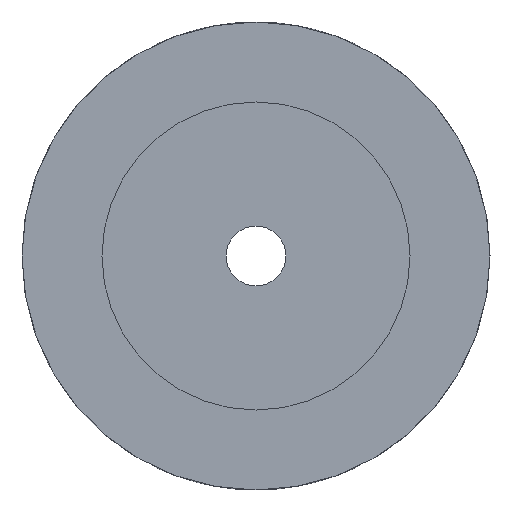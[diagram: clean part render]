
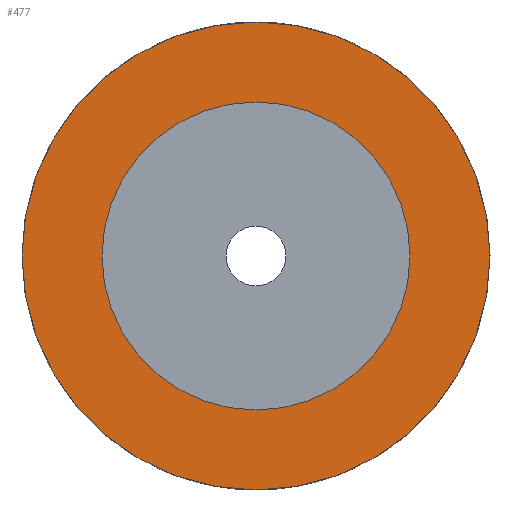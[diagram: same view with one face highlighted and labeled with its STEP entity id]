
A CAD part, front view. The second image highlights one B-rep face of the part: STEP entity #477.
In plain terms, the highlighted planar face has unit normal (0, -1, 0).
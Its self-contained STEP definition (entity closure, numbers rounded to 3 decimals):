
#27 = CARTESIAN_POINT ( 'NONE',  ( -2.625, 5.715, 0. ) ) ;
#30 = DIRECTION ( 'NONE',  ( -1., 0., 0. ) ) ;
#31 = DIRECTION ( 'NONE',  ( 0., 1., 0. ) ) ;
#33 = CARTESIAN_POINT ( 'NONE',  ( 0., 5.715, 0. ) ) ;
#34 = PLANE ( 'NONE',  #389 ) ;
#35 = CARTESIAN_POINT ( 'NONE',  ( 2.625, 5.715, 0. ) ) ;
#53 = CARTESIAN_POINT ( 'NONE',  ( -3.988, 5.715, 0. ) ) ;
#84 = DIRECTION ( 'NONE',  ( -1., 0., 0. ) ) ;
#85 = DIRECTION ( 'NONE',  ( 0., 1., 0. ) ) ;
#86 = CARTESIAN_POINT ( 'NONE',  ( 0., 5.715, 0. ) ) ;
#93 = DIRECTION ( 'NONE',  ( -1., 0., 0. ) ) ;
#94 = DIRECTION ( 'NONE',  ( 0., 1., 0. ) ) ;
#98 = CARTESIAN_POINT ( 'NONE',  ( 0., 5.715, 0. ) ) ;
#108 = DIRECTION ( 'NONE',  ( -1., 0., 0. ) ) ;
#109 = DIRECTION ( 'NONE',  ( 0., 1., 0. ) ) ;
#122 = CARTESIAN_POINT ( 'NONE',  ( 0., 5.715, 0. ) ) ;
#123 = DIRECTION ( 'NONE',  ( -1., 0., 0. ) ) ;
#124 = DIRECTION ( 'NONE',  ( 0., 1., 0. ) ) ;
#125 = CARTESIAN_POINT ( 'NONE',  ( 0., 5.715, 0. ) ) ;
#179 = CARTESIAN_POINT ( 'NONE',  ( 3.988, 5.715, 0. ) ) ;
#251 = EDGE_LOOP ( 'NONE', ( #320, #317 ) ) ;
#253 = EDGE_LOOP ( 'NONE', ( #314, #318 ) ) ;
#265 = VERTEX_POINT ( 'NONE', #53 ) ;
#273 = VERTEX_POINT ( 'NONE', #35 ) ;
#275 = VERTEX_POINT ( 'NONE', #27 ) ;
#278 = VERTEX_POINT ( 'NONE', #179 ) ;
#314 = ORIENTED_EDGE ( 'NONE', *, *, #494, .F. ) ;
#317 = ORIENTED_EDGE ( 'NONE', *, *, #507, .T. ) ;
#318 = ORIENTED_EDGE ( 'NONE', *, *, #499, .F. ) ;
#320 = ORIENTED_EDGE ( 'NONE', *, *, #504, .T. ) ;
#373 = AXIS2_PLACEMENT_3D ( 'NONE', #98, #94, #93 ) ;
#374 = AXIS2_PLACEMENT_3D ( 'NONE', #86, #85, #84 ) ;
#384 = AXIS2_PLACEMENT_3D ( 'NONE', #125, #124, #123 ) ;
#389 = AXIS2_PLACEMENT_3D ( 'NONE', #33, #31, #30 ) ;
#416 = FACE_BOUND ( 'NONE', #251, .T. ) ;
#434 = AXIS2_PLACEMENT_3D ( 'NONE', #122, #109, #108 ) ;
#441 = FACE_OUTER_BOUND ( 'NONE', #253, .T. ) ;
#460 = CIRCLE ( 'NONE', #374, 2.625 ) ;
#463 = CIRCLE ( 'NONE', #373, 2.625 ) ;
#467 = CIRCLE ( 'NONE', #434, 3.988 ) ;
#468 = CIRCLE ( 'NONE', #384, 3.988 ) ;
#477 = ADVANCED_FACE ( 'NONE', ( #441, #416 ), #34, .F. ) ;
#494 = EDGE_CURVE ( 'NONE', #265, #278, #468, .T. ) ;
#499 = EDGE_CURVE ( 'NONE', #278, #265, #467, .T. ) ;
#504 = EDGE_CURVE ( 'NONE', #275, #273, #463, .T. ) ;
#507 = EDGE_CURVE ( 'NONE', #273, #275, #460, .T. ) ;
